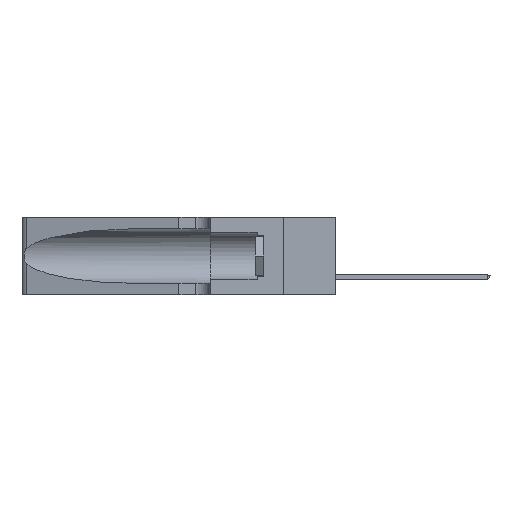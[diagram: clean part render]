
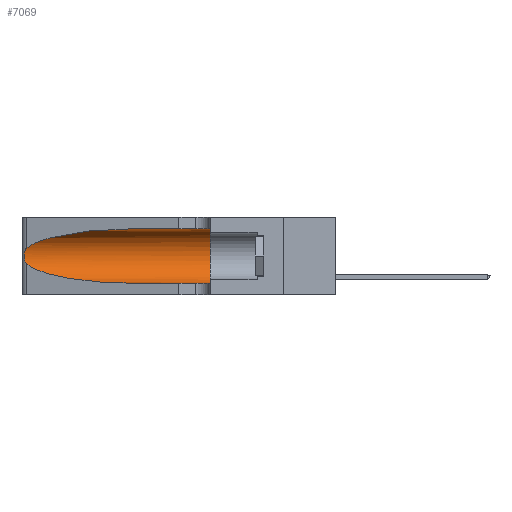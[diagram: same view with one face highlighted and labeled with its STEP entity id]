
A CAD part, left-side view. The second image highlights one B-rep face of the part: STEP entity #7069.
In plain terms, the highlighted cylindrical face has radius 3.308 mm (diameter 6.617 mm), a partial arc.
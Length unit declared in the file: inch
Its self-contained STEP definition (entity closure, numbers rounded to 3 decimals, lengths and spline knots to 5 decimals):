
#100 = EDGE_CURVE ( 'NONE', #1434, #13124, #14697, .T. ) ;
#357 = CARTESIAN_POINT ( 'NONE',  ( 0.18966, 0.96281, 0.31525 ) ) ;
#1042 = DIRECTION ( 'NONE',  ( 0., 1., 0. ) ) ;
#1306 = CARTESIAN_POINT ( 'NONE',  ( 0.25487, 1.22718, 0.14631 ) ) ;
#1359 = CARTESIAN_POINT ( 'NONE',  ( 0.25555, 1.22994, 0.2215 ) ) ;
#1434 = VERTEX_POINT ( 'NONE', #14100 ) ;
#1489 = DIRECTION ( 'NONE',  ( 0., -1., 0. ) ) ;
#2203 = ORIENTED_EDGE ( 'NONE', *, *, #18006, .T. ) ;
#2403 = CARTESIAN_POINT ( 'NONE',  ( 0.25487, 1.22718, 0.22369 ) ) ;
#2483 = CARTESIAN_POINT ( 'NONE',  ( 0.1305, 0.72297, 0.05475 ) ) ;
#2841 = LINE ( 'NONE', #15628, #21152 ) ;
#3127 = CARTESIAN_POINT ( 'NONE',  ( 0.26075, 1.23896, 0.178 ) ) ;
#3277 =( BOUNDED_CURVE ( )  B_SPLINE_CURVE ( 3, ( #22356, #357, #11277, #18514 ),
 .UNSPECIFIED., .F., .T. ) 
 B_SPLINE_CURVE_WITH_KNOTS ( ( 4, 4 ),
 ( 1.5708, 2.84003 ),
 .UNSPECIFIED. ) 
 CURVE ( )  GEOMETRIC_REPRESENTATION_ITEM ( )  RATIONAL_B_SPLINE_CURVE ( ( 1., 0.87, 0.87, 1. ) ) 
 REPRESENTATION_ITEM ( '' )  );
#3714 =( BOUNDED_CURVE ( )  B_SPLINE_CURVE ( 3, ( #18878, #4405, #6084, #2483 ),
 .UNSPECIFIED., .F., .F. ) 
 B_SPLINE_CURVE_WITH_KNOTS ( ( 4, 4 ),
 ( 3.44316, 4.71239 ),
 .UNSPECIFIED. ) 
 CURVE ( )  GEOMETRIC_REPRESENTATION_ITEM ( )  RATIONAL_B_SPLINE_CURVE ( ( 1., 0.87, 0.87, 1. ) ) 
 REPRESENTATION_ITEM ( '' )  );
#4405 = CARTESIAN_POINT ( 'NONE',  ( 0.2373, 1.15595, 0.08982 ) ) ;
#4688 = DIRECTION ( 'NONE',  ( 0., -1., 0. ) ) ;
#4745 = CARTESIAN_POINT ( 'NONE',  ( 0.25639, 1.23184, 0.21858 ) ) ;
#4752 = B_SPLINE_CURVE_WITH_KNOTS ( 'NONE', 3,
 ( #19458, #1359, #4745, #19689, #19380, #14184, #15844, #3127, #8415, #19540, #21207, #15769, #4819, #17598 ),
 .UNSPECIFIED., .F., .F.,
 ( 4, 2, 2, 2, 2, 2, 4 ),
 ( 0., 0.00027, 0.00053, 0.00107, 0.0016, 0.00187, 0.00214 ),
 .UNSPECIFIED. ) ;
#4819 = CARTESIAN_POINT ( 'NONE',  ( 0.25555, 1.22993, 0.14849 ) ) ;
#4872 = EDGE_LOOP ( 'NONE', ( #8876, #2203, #8838, #20022, #14984, #14582 ) ) ;
#5015 = CARTESIAN_POINT ( 'NONE',  ( 0.1305, 1.61858, 0.185 ) ) ;
#5290 = CYLINDRICAL_SURFACE ( 'NONE', #16438, 0.13025 ) ;
#5913 = CARTESIAN_POINT ( 'NONE',  ( 0.1305, 0.35, 0.05475 ) ) ;
#6084 = CARTESIAN_POINT ( 'NONE',  ( 0.18966, 0.96281, 0.05475 ) ) ;
#6157 = CARTESIAN_POINT ( 'NONE',  ( 0.1305, 0.72297, 0.31525 ) ) ;
#6452 = FACE_OUTER_BOUND ( 'NONE', #4872, .T. ) ;
#7069 = ADVANCED_FACE ( 'NONE', ( #6452 ), #5290, .F. ) ;
#7098 = DIRECTION ( 'NONE',  ( 0., 0., -1. ) ) ;
#7844 = DIRECTION ( 'NONE',  ( 0., -1., 0. ) ) ;
#8415 = CARTESIAN_POINT ( 'NONE',  ( 0.26017, 1.23833, 0.17102 ) ) ;
#8838 = ORIENTED_EDGE ( 'NONE', *, *, #18291, .T. ) ;
#8876 = ORIENTED_EDGE ( 'NONE', *, *, #17084, .T. ) ;
#8984 = AXIS2_PLACEMENT_3D ( 'NONE', #12029, #1042, #15686 ) ;
#9440 = CARTESIAN_POINT ( 'NONE',  ( 0.1305, 1.61858, 0.05475 ) ) ;
#9717 = EDGE_CURVE ( 'NONE', #18375, #1434, #2841, .T. ) ;
#10842 = CARTESIAN_POINT ( 'NONE',  ( 0.1305, 0.72297, 0.05475 ) ) ;
#11277 = CARTESIAN_POINT ( 'NONE',  ( 0.2373, 1.15595, 0.28018 ) ) ;
#12029 = CARTESIAN_POINT ( 'NONE',  ( 0.1305, 0.35, 0.185 ) ) ;
#12176 = VERTEX_POINT ( 'NONE', #10842 ) ;
#13124 = VERTEX_POINT ( 'NONE', #5913 ) ;
#14100 = CARTESIAN_POINT ( 'NONE',  ( 0.1305, 0.35, 0.31525 ) ) ;
#14184 = CARTESIAN_POINT ( 'NONE',  ( 0.26018, 1.23835, 0.19895 ) ) ;
#14582 = ORIENTED_EDGE ( 'NONE', *, *, #9717, .F. ) ;
#14697 = CIRCLE ( 'NONE', #8984, 0.13025 ) ;
#14984 = ORIENTED_EDGE ( 'NONE', *, *, #100, .F. ) ;
#15628 = CARTESIAN_POINT ( 'NONE',  ( 0.1305, 1.61858, 0.31525 ) ) ;
#15686 = DIRECTION ( 'NONE',  ( 0., 0., 1. ) ) ;
#15769 = CARTESIAN_POINT ( 'NONE',  ( 0.25639, 1.23186, 0.15144 ) ) ;
#15844 = CARTESIAN_POINT ( 'NONE',  ( 0.26075, 1.23896, 0.19203 ) ) ;
#16438 = AXIS2_PLACEMENT_3D ( 'NONE', #5015, #1489, #7098 ) ;
#17084 = EDGE_CURVE ( 'NONE', #18375, #18363, #3277, .T. ) ;
#17598 = CARTESIAN_POINT ( 'NONE',  ( 0.25487, 1.22718, 0.14631 ) ) ;
#18006 = EDGE_CURVE ( 'NONE', #18363, #21415, #4752, .T. ) ;
#18291 = EDGE_CURVE ( 'NONE', #21415, #12176, #3714, .T. ) ;
#18363 = VERTEX_POINT ( 'NONE', #2403 ) ;
#18375 = VERTEX_POINT ( 'NONE', #6157 ) ;
#18514 = CARTESIAN_POINT ( 'NONE',  ( 0.25487, 1.22718, 0.22369 ) ) ;
#18878 = CARTESIAN_POINT ( 'NONE',  ( 0.25487, 1.22718, 0.14631 ) ) ;
#19380 = CARTESIAN_POINT ( 'NONE',  ( 0.25854, 1.2359, 0.20912 ) ) ;
#19458 = CARTESIAN_POINT ( 'NONE',  ( 0.25487, 1.22718, 0.22369 ) ) ;
#19540 = CARTESIAN_POINT ( 'NONE',  ( 0.25856, 1.23593, 0.16098 ) ) ;
#19689 = CARTESIAN_POINT ( 'NONE',  ( 0.25787, 1.23484, 0.2124 ) ) ;
#20022 = ORIENTED_EDGE ( 'NONE', *, *, #23589, .T. ) ;
#21152 = VECTOR ( 'NONE', #4688, 39.37008 ) ;
#21207 = CARTESIAN_POINT ( 'NONE',  ( 0.25789, 1.23486, 0.15765 ) ) ;
#21415 = VERTEX_POINT ( 'NONE', #1306 ) ;
#21594 = VECTOR ( 'NONE', #7844, 39.37008 ) ;
#22171 = LINE ( 'NONE', #9440, #21594 ) ;
#22356 = CARTESIAN_POINT ( 'NONE',  ( 0.1305, 0.72297, 0.31525 ) ) ;
#23589 = EDGE_CURVE ( 'NONE', #12176, #13124, #22171, .T. ) ;
